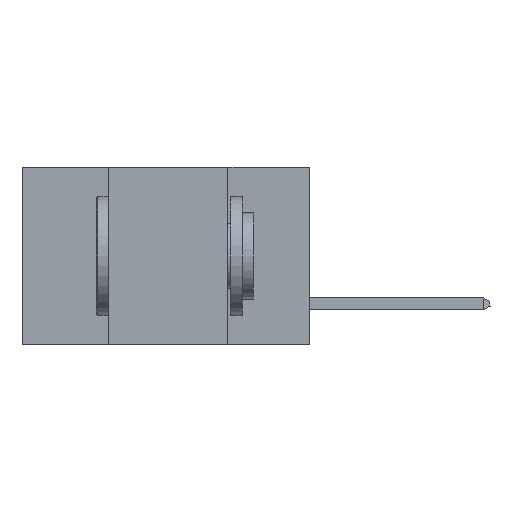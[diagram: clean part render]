
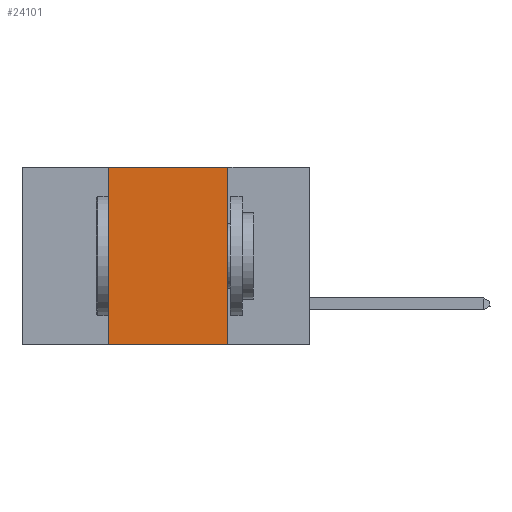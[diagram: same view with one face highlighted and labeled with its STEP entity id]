
A CAD part, left-side view. The second image highlights one B-rep face of the part: STEP entity #24101.
In plain terms, the highlighted planar face has unit normal (-1, 0, 0).
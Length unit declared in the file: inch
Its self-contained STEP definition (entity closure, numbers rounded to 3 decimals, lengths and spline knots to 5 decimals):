
#371 = AXIS2_PLACEMENT_3D ( 'NONE', #23497, #16187, #21004 ) ;
#1603 = ORIENTED_EDGE ( 'NONE', *, *, #5403, .F. ) ;
#2737 = DIRECTION ( 'NONE',  ( 0., -1., 0. ) ) ;
#3959 = CARTESIAN_POINT ( 'NONE',  ( 0., 0.6, -0.37 ) ) ;
#4474 = ORIENTED_EDGE ( 'NONE', *, *, #32545, .F. ) ;
#5403 = EDGE_CURVE ( 'NONE', #33043, #30009, #22472, .T. ) ;
#5786 = LINE ( 'NONE', #14359, #14360 ) ;
#6454 = VERTEX_POINT ( 'NONE', #11247 ) ;
#6558 = ORIENTED_EDGE ( 'NONE', *, *, #31733, .T. ) ;
#7747 = ORIENTED_EDGE ( 'NONE', *, *, #24779, .F. ) ;
#8238 = FACE_OUTER_BOUND ( 'NONE', #10606, .T. ) ;
#8776 = CARTESIAN_POINT ( 'NONE',  ( 0., 0.42, 0. ) ) ;
#9430 = VECTOR ( 'NONE', #33478, 39.37008 ) ;
#10606 = EDGE_LOOP ( 'NONE', ( #4474, #7747, #1603, #6558 ) ) ;
#11120 = LINE ( 'NONE', #3959, #17648 ) ;
#11247 = CARTESIAN_POINT ( 'NONE',  ( 0., 0.17, -0.37 ) ) ;
#13112 = LINE ( 'NONE', #30970, #20478 ) ;
#14359 = CARTESIAN_POINT ( 'NONE',  ( 0., 0.6, 0. ) ) ;
#14360 = VECTOR ( 'NONE', #2737, 39.37008 ) ;
#16187 = DIRECTION ( 'NONE',  ( 1., 0., 0. ) ) ;
#17648 = VECTOR ( 'NONE', #22157, 39.37008 ) ;
#17998 = CARTESIAN_POINT ( 'NONE',  ( 0., 0.42, 0. ) ) ;
#20212 = VERTEX_POINT ( 'NONE', #23073 ) ;
#20478 = VECTOR ( 'NONE', #23224, 39.37008 ) ;
#21004 = DIRECTION ( 'NONE',  ( 0., 0., -1. ) ) ;
#22157 = DIRECTION ( 'NONE',  ( 0., -1., 0. ) ) ;
#22472 = LINE ( 'NONE', #17998, #9430 ) ;
#23073 = CARTESIAN_POINT ( 'NONE',  ( 0., 0.17, 0. ) ) ;
#23224 = DIRECTION ( 'NONE',  ( 0., 0., -1. ) ) ;
#23497 = CARTESIAN_POINT ( 'NONE',  ( 0., 0.6, 0. ) ) ;
#24101 = ADVANCED_FACE ( 'NONE', ( #8238 ), #31228, .F. ) ;
#24779 = EDGE_CURVE ( 'NONE', #30009, #20212, #5786, .T. ) ;
#30009 = VERTEX_POINT ( 'NONE', #8776 ) ;
#30970 = CARTESIAN_POINT ( 'NONE',  ( 0., 0.17, 0. ) ) ;
#31228 = PLANE ( 'NONE',  #371 ) ;
#31733 = EDGE_CURVE ( 'NONE', #33043, #6454, #11120, .T. ) ;
#32545 = EDGE_CURVE ( 'NONE', #20212, #6454, #13112, .T. ) ;
#33043 = VERTEX_POINT ( 'NONE', #33644 ) ;
#33478 = DIRECTION ( 'NONE',  ( 0., 0., 1. ) ) ;
#33644 = CARTESIAN_POINT ( 'NONE',  ( 0., 0.42, -0.37 ) ) ;
